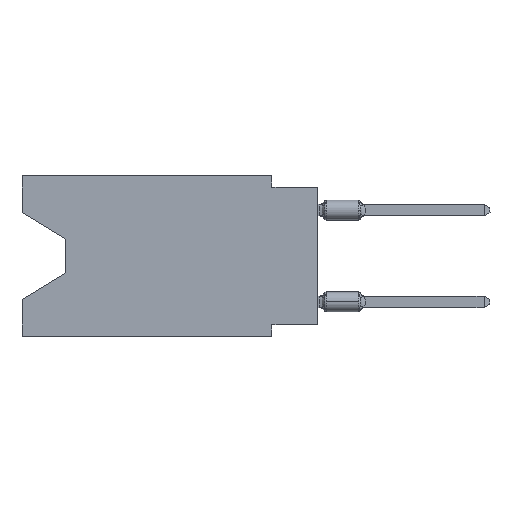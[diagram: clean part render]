
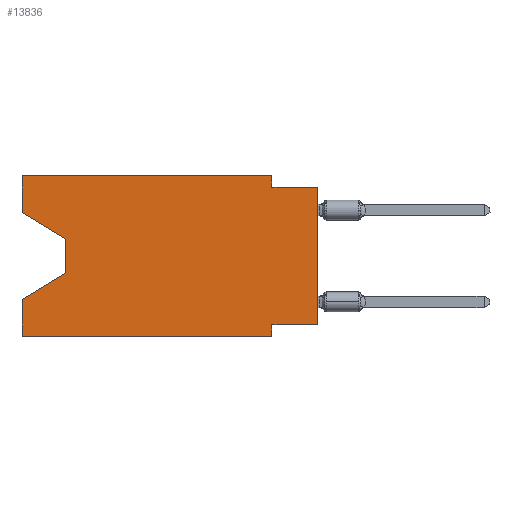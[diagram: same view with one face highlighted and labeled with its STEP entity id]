
A CAD part, left-side view. The second image highlights one B-rep face of the part: STEP entity #13836.
In plain terms, the highlighted planar face has unit normal (-1, 0, 0).
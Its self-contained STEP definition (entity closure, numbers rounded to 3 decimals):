
#251 = EDGE_LOOP ( 'NONE', ( #576, #12875, #8584, #14497, #12174, #5893, #15666, #1104, #7712, #8241, #9631, #2299 ) ) ;
#269 = VERTEX_POINT ( 'NONE', #13356 ) ;
#548 = CARTESIAN_POINT ( 'NONE',  ( 0., 2.54, -8.89 ) ) ;
#563 = CARTESIAN_POINT ( 'NONE',  ( 0., 2.54, 0. ) ) ;
#576 = ORIENTED_EDGE ( 'NONE', *, *, #14395, .T. ) ;
#833 = DIRECTION ( 'NONE',  ( 0., -1., 0. ) ) ;
#880 = CARTESIAN_POINT ( 'NONE',  ( 0., 16.383, 0. ) ) ;
#1104 = ORIENTED_EDGE ( 'NONE', *, *, #7097, .T. ) ;
#1161 = CARTESIAN_POINT ( 'NONE',  ( 0., 0., -8.255 ) ) ;
#1203 = LINE ( 'NONE', #3885, #5999 ) ;
#1766 = DIRECTION ( 'NONE',  ( 0., 1., 0. ) ) ;
#1848 = CARTESIAN_POINT ( 'NONE',  ( 0., 0., -0.635 ) ) ;
#2299 = ORIENTED_EDGE ( 'NONE', *, *, #7906, .F. ) ;
#2411 = DIRECTION ( 'NONE',  ( 1., 0., 0. ) ) ;
#2462 = VECTOR ( 'NONE', #9200, 1000. ) ;
#2958 = VERTEX_POINT ( 'NONE', #14130 ) ;
#2974 = VERTEX_POINT ( 'NONE', #7750 ) ;
#3081 = EDGE_CURVE ( 'NONE', #269, #4056, #11771, .T. ) ;
#3163 = LINE ( 'NONE', #880, #8175 ) ;
#3257 = EDGE_CURVE ( 'NONE', #8812, #14923, #13518, .T. ) ;
#3428 = LINE ( 'NONE', #13277, #11632 ) ;
#3589 = PLANE ( 'NONE',  #5198 ) ;
#3885 = CARTESIAN_POINT ( 'NONE',  ( 0., 13.97, -5.385 ) ) ;
#4056 = VERTEX_POINT ( 'NONE', #548 ) ;
#4144 = VECTOR ( 'NONE', #9524, 1000. ) ;
#4527 = VECTOR ( 'NONE', #833, 1000. ) ;
#4784 = LINE ( 'NONE', #7317, #8116 ) ;
#5068 = DIRECTION ( 'NONE',  ( 0., 0., 1. ) ) ;
#5198 = AXIS2_PLACEMENT_3D ( 'NONE', #8735, #2411, #11728 ) ;
#5801 = CARTESIAN_POINT ( 'NONE',  ( 0., 13.97, -3.505 ) ) ;
#5862 = DIRECTION ( 'NONE',  ( 0., 0., 1. ) ) ;
#5893 = ORIENTED_EDGE ( 'NONE', *, *, #14595, .F. ) ;
#5999 = VECTOR ( 'NONE', #6234, 1000. ) ;
#6007 = VERTEX_POINT ( 'NONE', #7036 ) ;
#6011 = EDGE_CURVE ( 'NONE', #12330, #8812, #9343, .T. ) ;
#6234 = DIRECTION ( 'NONE',  ( 0., 0.855, -0.519 ) ) ;
#6278 = FACE_OUTER_BOUND ( 'NONE', #251, .T. ) ;
#6350 = CARTESIAN_POINT ( 'NONE',  ( 0., 16.383, -2.038 ) ) ;
#6528 = EDGE_CURVE ( 'NONE', #2974, #12330, #3163, .T. ) ;
#6735 = CARTESIAN_POINT ( 'NONE',  ( 0., 16.383, -2.038 ) ) ;
#7036 = CARTESIAN_POINT ( 'NONE',  ( 0., 13.97, -3.505 ) ) ;
#7097 = EDGE_CURVE ( 'NONE', #12241, #14923, #12798, .T. ) ;
#7317 = CARTESIAN_POINT ( 'NONE',  ( 0., 2.54, -8.89 ) ) ;
#7712 = ORIENTED_EDGE ( 'NONE', *, *, #3257, .F. ) ;
#7750 = CARTESIAN_POINT ( 'NONE',  ( 0., 16.383, 0. ) ) ;
#7906 = EDGE_CURVE ( 'NONE', #11393, #2974, #16511, .T. ) ;
#8090 = LINE ( 'NONE', #6735, #2462 ) ;
#8116 = VECTOR ( 'NONE', #11100, 1000. ) ;
#8175 = VECTOR ( 'NONE', #13487, 1000. ) ;
#8241 = ORIENTED_EDGE ( 'NONE', *, *, #6011, .F. ) ;
#8366 = VECTOR ( 'NONE', #14444, 1000. ) ;
#8584 = ORIENTED_EDGE ( 'NONE', *, *, #9421, .T. ) ;
#8589 = EDGE_CURVE ( 'NONE', #6007, #13334, #9611, .T. ) ;
#8735 = CARTESIAN_POINT ( 'NONE',  ( 0., 16.383, 0. ) ) ;
#8812 = VERTEX_POINT ( 'NONE', #14279 ) ;
#9004 = EDGE_CURVE ( 'NONE', #12241, #13133, #3428, .T. ) ;
#9200 = DIRECTION ( 'NONE',  ( 0., -0.855, -0.519 ) ) ;
#9343 = LINE ( 'NONE', #563, #8366 ) ;
#9421 = EDGE_CURVE ( 'NONE', #13334, #2958, #1203, .T. ) ;
#9524 = DIRECTION ( 'NONE',  ( 0., 0., -1. ) ) ;
#9611 = LINE ( 'NONE', #5801, #4144 ) ;
#9631 = ORIENTED_EDGE ( 'NONE', *, *, #6528, .F. ) ;
#10134 = CARTESIAN_POINT ( 'NONE',  ( 0., 2.54, -8.255 ) ) ;
#10832 = LINE ( 'NONE', #15949, #14846 ) ;
#11100 = DIRECTION ( 'NONE',  ( 0., 0., -1. ) ) ;
#11251 = CARTESIAN_POINT ( 'NONE',  ( 0., 2.54, 0. ) ) ;
#11393 = VERTEX_POINT ( 'NONE', #6350 ) ;
#11632 = VECTOR ( 'NONE', #1766, 1000. ) ;
#11728 = DIRECTION ( 'NONE',  ( 0., 0., -1. ) ) ;
#11771 = LINE ( 'NONE', #14290, #13139 ) ;
#12174 = ORIENTED_EDGE ( 'NONE', *, *, #3081, .T. ) ;
#12241 = VERTEX_POINT ( 'NONE', #1161 ) ;
#12330 = VERTEX_POINT ( 'NONE', #11251 ) ;
#12798 = LINE ( 'NONE', #14139, #15431 ) ;
#12875 = ORIENTED_EDGE ( 'NONE', *, *, #8589, .T. ) ;
#13133 = VERTEX_POINT ( 'NONE', #10134 ) ;
#13139 = VECTOR ( 'NONE', #14211, 1000. ) ;
#13277 = CARTESIAN_POINT ( 'NONE',  ( 0., 0., -8.255 ) ) ;
#13334 = VERTEX_POINT ( 'NONE', #15503 ) ;
#13356 = CARTESIAN_POINT ( 'NONE',  ( 0., 16.383, -8.89 ) ) ;
#13487 = DIRECTION ( 'NONE',  ( 0., -1., 0. ) ) ;
#13518 = LINE ( 'NONE', #1848, #4527 ) ;
#13836 = ADVANCED_FACE ( 'NONE', ( #6278 ), #3589, .F. ) ;
#13967 = DIRECTION ( 'NONE',  ( 0., 0., 1. ) ) ;
#14130 = CARTESIAN_POINT ( 'NONE',  ( 0., 16.383, -6.852 ) ) ;
#14139 = CARTESIAN_POINT ( 'NONE',  ( 0., 0., 0. ) ) ;
#14211 = DIRECTION ( 'NONE',  ( 0., -1., 0. ) ) ;
#14279 = CARTESIAN_POINT ( 'NONE',  ( 0., 2.54, -0.635 ) ) ;
#14290 = CARTESIAN_POINT ( 'NONE',  ( 0., 16.383, -8.89 ) ) ;
#14395 = EDGE_CURVE ( 'NONE', #11393, #6007, #8090, .T. ) ;
#14444 = DIRECTION ( 'NONE',  ( 0., 0., -1. ) ) ;
#14497 = ORIENTED_EDGE ( 'NONE', *, *, #15001, .F. ) ;
#14595 = EDGE_CURVE ( 'NONE', #13133, #4056, #4784, .T. ) ;
#14846 = VECTOR ( 'NONE', #5862, 1000. ) ;
#14912 = VECTOR ( 'NONE', #5068, 1000. ) ;
#14923 = VERTEX_POINT ( 'NONE', #15793 ) ;
#15001 = EDGE_CURVE ( 'NONE', #269, #2958, #10832, .T. ) ;
#15259 = CARTESIAN_POINT ( 'NONE',  ( 0., 16.383, 0. ) ) ;
#15431 = VECTOR ( 'NONE', #13967, 1000. ) ;
#15503 = CARTESIAN_POINT ( 'NONE',  ( 0., 13.97, -5.385 ) ) ;
#15666 = ORIENTED_EDGE ( 'NONE', *, *, #9004, .F. ) ;
#15793 = CARTESIAN_POINT ( 'NONE',  ( 0., 0., -0.635 ) ) ;
#15949 = CARTESIAN_POINT ( 'NONE',  ( 0., 16.383, 0. ) ) ;
#16511 = LINE ( 'NONE', #15259, #14912 ) ;
